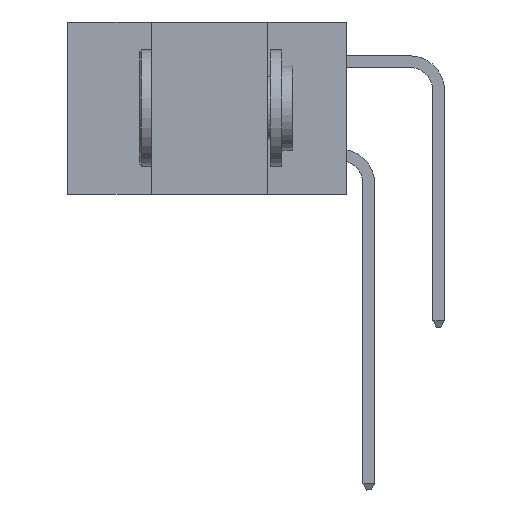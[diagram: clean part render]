
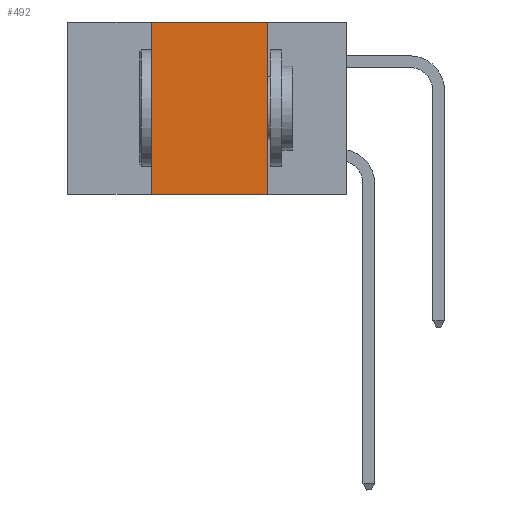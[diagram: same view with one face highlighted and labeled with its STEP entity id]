
A CAD part, left-side view. The second image highlights one B-rep face of the part: STEP entity #492.
In plain terms, the highlighted planar face has unit normal (-1, 0, 0).
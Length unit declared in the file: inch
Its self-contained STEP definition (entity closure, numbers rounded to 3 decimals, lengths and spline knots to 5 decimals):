
#282 = CARTESIAN_POINT ( 'NONE',  ( 0., 0.6, 0. ) ) ;
#492 = ADVANCED_FACE ( 'NONE', ( #6228 ), #5138, .F. ) ;
#570 = VECTOR ( 'NONE', #3082, 39.37008 ) ;
#1199 = EDGE_CURVE ( 'NONE', #2363, #7642, #7943, .T. ) ;
#1828 = VERTEX_POINT ( 'NONE', #4458 ) ;
#1964 = VERTEX_POINT ( 'NONE', #10216 ) ;
#2004 = EDGE_CURVE ( 'NONE', #1828, #1964, #3012, .T. ) ;
#2323 = DIRECTION ( 'NONE',  ( 0., 0., -1. ) ) ;
#2363 = VERTEX_POINT ( 'NONE', #3398 ) ;
#3012 = LINE ( 'NONE', #282, #570 ) ;
#3082 = DIRECTION ( 'NONE',  ( 0., -1., 0. ) ) ;
#3398 = CARTESIAN_POINT ( 'NONE',  ( 0., 0.42, -0.37 ) ) ;
#3596 = VECTOR ( 'NONE', #8837, 39.37008 ) ;
#4001 = DIRECTION ( 'NONE',  ( 0., 0., -1. ) ) ;
#4173 = EDGE_CURVE ( 'NONE', #2363, #1828, #5701, .T. ) ;
#4354 = CARTESIAN_POINT ( 'NONE',  ( 0., 0.17, -0.37 ) ) ;
#4458 = CARTESIAN_POINT ( 'NONE',  ( 0., 0.42, 0. ) ) ;
#4973 = VECTOR ( 'NONE', #7179, 39.37008 ) ;
#5105 = CARTESIAN_POINT ( 'NONE',  ( 0., 0.6, 0. ) ) ;
#5138 = PLANE ( 'NONE',  #10525 ) ;
#5671 = ORIENTED_EDGE ( 'NONE', *, *, #4173, .F. ) ;
#5701 = LINE ( 'NONE', #6252, #4973 ) ;
#5778 = VECTOR ( 'NONE', #4001, 39.37008 ) ;
#6104 = ORIENTED_EDGE ( 'NONE', *, *, #1199, .T. ) ;
#6228 = FACE_OUTER_BOUND ( 'NONE', #10609, .T. ) ;
#6252 = CARTESIAN_POINT ( 'NONE',  ( 0., 0.42, 0. ) ) ;
#6538 = ORIENTED_EDGE ( 'NONE', *, *, #2004, .F. ) ;
#6991 = DIRECTION ( 'NONE',  ( 1., 0., 0. ) ) ;
#7179 = DIRECTION ( 'NONE',  ( 0., 0., 1. ) ) ;
#7642 = VERTEX_POINT ( 'NONE', #4354 ) ;
#7853 = ORIENTED_EDGE ( 'NONE', *, *, #9813, .F. ) ;
#7943 = LINE ( 'NONE', #8988, #3596 ) ;
#8837 = DIRECTION ( 'NONE',  ( 0., -1., 0. ) ) ;
#8988 = CARTESIAN_POINT ( 'NONE',  ( 0., 0.6, -0.37 ) ) ;
#9411 = LINE ( 'NONE', #9997, #5778 ) ;
#9813 = EDGE_CURVE ( 'NONE', #1964, #7642, #9411, .T. ) ;
#9997 = CARTESIAN_POINT ( 'NONE',  ( 0., 0.17, 0. ) ) ;
#10216 = CARTESIAN_POINT ( 'NONE',  ( 0., 0.17, 0. ) ) ;
#10525 = AXIS2_PLACEMENT_3D ( 'NONE', #5105, #6991, #2323 ) ;
#10609 = EDGE_LOOP ( 'NONE', ( #7853, #6538, #5671, #6104 ) ) ;
